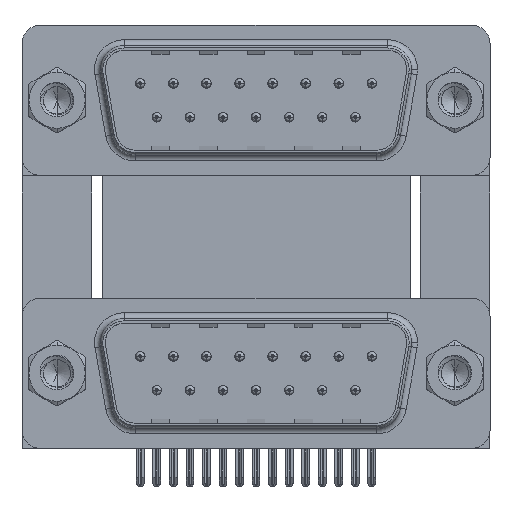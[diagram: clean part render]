
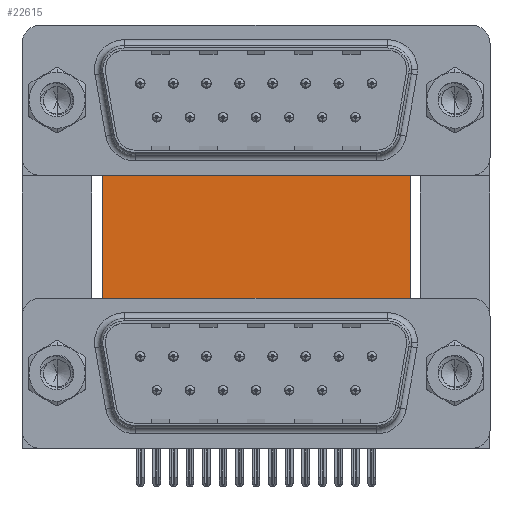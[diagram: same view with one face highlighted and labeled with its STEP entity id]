
A CAD part, top view. The second image highlights one B-rep face of the part: STEP entity #22615.
In plain terms, the highlighted planar face has unit normal (0, 0, 1).
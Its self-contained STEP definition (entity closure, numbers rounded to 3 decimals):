
#198 = EDGE_CURVE ( 'NONE', #9091, #14303, #9356, .T. ) ;
#2267 = LINE ( 'NONE', #38457, #21761 ) ;
#3323 = PLANE ( 'NONE',  #22876 ) ;
#4042 = DIRECTION ( 'NONE',  ( 0., -1., 0. ) ) ;
#5731 = ORIENTED_EDGE ( 'NONE', *, *, #6294, .T. ) ;
#6294 = EDGE_CURVE ( 'NONE', #31543, #14199, #19332, .T. ) ;
#7242 = CARTESIAN_POINT ( 'NONE',  ( 3.79, 16.585, -12. ) ) ;
#7807 = DIRECTION ( 'NONE',  ( 0., -1., 0. ) ) ;
#8242 = CARTESIAN_POINT ( 'NONE',  ( 3.79, -3.735, -12. ) ) ;
#9091 = VERTEX_POINT ( 'NONE', #24848 ) ;
#9356 = LINE ( 'NONE', #21264, #14174 ) ;
#10340 = EDGE_CURVE ( 'NONE', #14199, #14303, #11582, .T. ) ;
#11582 = LINE ( 'NONE', #32927, #16647 ) ;
#14174 = VECTOR ( 'NONE', #4042, 1000. ) ;
#14199 = VERTEX_POINT ( 'NONE', #8242 ) ;
#14303 = VERTEX_POINT ( 'NONE', #18155 ) ;
#15221 = DIRECTION ( 'NONE',  ( -1., 0., 0. ) ) ;
#16647 = VECTOR ( 'NONE', #30000, 1000. ) ;
#18155 = CARTESIAN_POINT ( 'NONE',  ( 29.58, -3.735, -12. ) ) ;
#19332 = LINE ( 'NONE', #7242, #36569 ) ;
#21264 = CARTESIAN_POINT ( 'NONE',  ( 29.58, 16.585, -12. ) ) ;
#21761 = VECTOR ( 'NONE', #32615, 1000. ) ;
#22615 = ADVANCED_FACE ( 'NONE', ( #24811 ), #3323, .F. ) ;
#22876 = AXIS2_PLACEMENT_3D ( 'NONE', #33652, #27590, #15221 ) ;
#24811 = FACE_OUTER_BOUND ( 'NONE', #26929, .T. ) ;
#24848 = CARTESIAN_POINT ( 'NONE',  ( 29.58, 16.585, -12. ) ) ;
#26929 = EDGE_LOOP ( 'NONE', ( #28669, #33819, #27715, #5731 ) ) ;
#27590 = DIRECTION ( 'NONE',  ( 0., 0., -1. ) ) ;
#27715 = ORIENTED_EDGE ( 'NONE', *, *, #31905, .F. ) ;
#28669 = ORIENTED_EDGE ( 'NONE', *, *, #10340, .T. ) ;
#29451 = CARTESIAN_POINT ( 'NONE',  ( 3.79, 16.585, -12. ) ) ;
#30000 = DIRECTION ( 'NONE',  ( 1., 0., 0. ) ) ;
#31543 = VERTEX_POINT ( 'NONE', #29451 ) ;
#31905 = EDGE_CURVE ( 'NONE', #31543, #9091, #2267, .T. ) ;
#32615 = DIRECTION ( 'NONE',  ( 1., 0., 0. ) ) ;
#32927 = CARTESIAN_POINT ( 'NONE',  ( 3.79, -3.735, -12. ) ) ;
#33652 = CARTESIAN_POINT ( 'NONE',  ( 3.79, 16.585, -12. ) ) ;
#33819 = ORIENTED_EDGE ( 'NONE', *, *, #198, .F. ) ;
#36569 = VECTOR ( 'NONE', #7807, 1000. ) ;
#38457 = CARTESIAN_POINT ( 'NONE',  ( 3.79, 16.585, -12. ) ) ;
